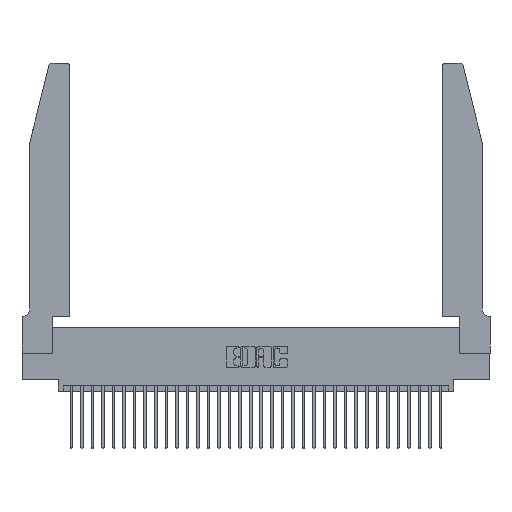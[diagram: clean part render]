
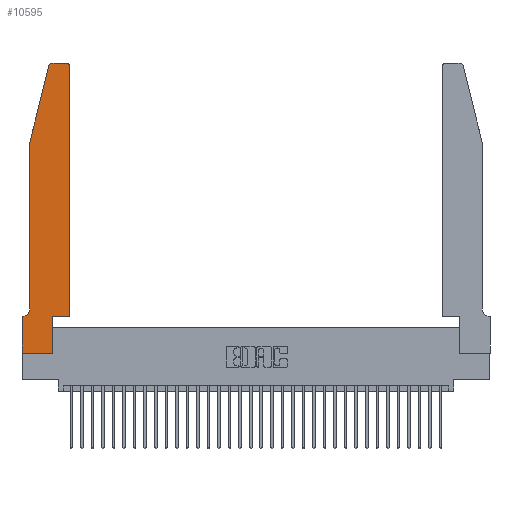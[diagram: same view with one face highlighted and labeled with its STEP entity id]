
A CAD part, top view. The second image highlights one B-rep face of the part: STEP entity #10595.
In plain terms, the highlighted planar face has unit normal (0, 0, 1).
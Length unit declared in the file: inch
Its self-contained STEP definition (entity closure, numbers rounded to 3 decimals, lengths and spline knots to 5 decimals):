
#667 = DIRECTION ( 'NONE',  ( 1., 0., 0. ) ) ;
#1403 = EDGE_CURVE ( 'NONE', #10720, #30104, #23842, .T. ) ;
#1773 = CARTESIAN_POINT ( 'NONE',  ( 0.0055, 0.42, 0.37 ) ) ;
#1906 = VERTEX_POINT ( 'NONE', #26110 ) ;
#2204 = LINE ( 'NONE', #24118, #9197 ) ;
#2300 = ORIENTED_EDGE ( 'NONE', *, *, #12533, .T. ) ;
#2675 = DIRECTION ( 'NONE',  ( 0., 0., 1. ) ) ;
#2886 = ORIENTED_EDGE ( 'NONE', *, *, #8794, .T. ) ;
#3018 = ORIENTED_EDGE ( 'NONE', *, *, #29753, .T. ) ;
#3144 = DIRECTION ( 'NONE',  ( -0.239, -0.971, 0. ) ) ;
#3188 = CIRCLE ( 'NONE', #26327, 0.03 ) ;
#3251 = ORIENTED_EDGE ( 'NONE', *, *, #10801, .T. ) ;
#3457 = VERTEX_POINT ( 'NONE', #25973 ) ;
#4289 = LINE ( 'NONE', #22134, #23551 ) ;
#4416 = DIRECTION ( 'NONE',  ( -1., 0., 0. ) ) ;
#4576 = VECTOR ( 'NONE', #12231, 39.37008 ) ;
#5219 = CARTESIAN_POINT ( 'NONE',  ( 0.4205, 2.75, 0.37 ) ) ;
#5994 = CARTESIAN_POINT ( 'NONE',  ( 0.0755, 0.35, 0.37 ) ) ;
#6241 = EDGE_CURVE ( 'NONE', #12046, #10720, #6479, .T. ) ;
#6479 = LINE ( 'NONE', #24213, #26583 ) ;
#6564 = CARTESIAN_POINT ( 'NONE',  ( 0.4505, 2.72, 0.37 ) ) ;
#6740 = CARTESIAN_POINT ( 'NONE',  ( 0.2865, 0.35, 0.37 ) ) ;
#8004 = LINE ( 'NONE', #16679, #20241 ) ;
#8794 = EDGE_CURVE ( 'NONE', #32573, #12046, #8004, .T. ) ;
#8843 = VECTOR ( 'NONE', #13750, 39.37008 ) ;
#8934 = DIRECTION ( 'NONE',  ( 1., 0., 0. ) ) ;
#9123 = VERTEX_POINT ( 'NONE', #21591 ) ;
#9197 = VECTOR ( 'NONE', #3144, 39.37008 ) ;
#9955 = CARTESIAN_POINT ( 'NONE',  ( 0., 0.35, 0.37 ) ) ;
#10167 = CARTESIAN_POINT ( 'NONE',  ( 0., 0., 0.37 ) ) ;
#10417 = CARTESIAN_POINT ( 'NONE',  ( 0.4505, 0.35, 0.37 ) ) ;
#10595 = ADVANCED_FACE ( 'NONE', ( #31246 ), #19295, .T. ) ;
#10720 = VERTEX_POINT ( 'NONE', #11905 ) ;
#10722 = LINE ( 'NONE', #30584, #4576 ) ;
#10801 = EDGE_CURVE ( 'NONE', #33140, #3457, #10722, .T. ) ;
#11279 = VERTEX_POINT ( 'NONE', #32528 ) ;
#11442 = DIRECTION ( 'NONE',  ( 0., 1., 0. ) ) ;
#11887 = VECTOR ( 'NONE', #17566, 39.37008 ) ;
#11905 = CARTESIAN_POINT ( 'NONE',  ( 0.4505, 0.35, 0.37 ) ) ;
#12046 = VERTEX_POINT ( 'NONE', #6740 ) ;
#12231 = DIRECTION ( 'NONE',  ( -1., 0., 0. ) ) ;
#12533 = EDGE_CURVE ( 'NONE', #29848, #1906, #2204, .T. ) ;
#13750 = DIRECTION ( 'NONE',  ( 0., -1., 0. ) ) ;
#14697 = ORIENTED_EDGE ( 'NONE', *, *, #17729, .T. ) ;
#14990 = EDGE_CURVE ( 'NONE', #1906, #9123, #32786, .T. ) ;
#15049 = DIRECTION ( 'NONE',  ( 0., 1., 0. ) ) ;
#15271 = DIRECTION ( 'NONE',  ( 0., 0., 1. ) ) ;
#15705 = AXIS2_PLACEMENT_3D ( 'NONE', #32400, #24634, #8934 ) ;
#16019 = VECTOR ( 'NONE', #15049, 39.37008 ) ;
#16679 = CARTESIAN_POINT ( 'NONE',  ( 0.2865, 0.35, 0.37 ) ) ;
#16908 = ORIENTED_EDGE ( 'NONE', *, *, #6241, .T. ) ;
#17566 = DIRECTION ( 'NONE',  ( 0., -1., 0. ) ) ;
#17729 = EDGE_CURVE ( 'NONE', #3457, #29848, #29972, .T. ) ;
#17796 = ORIENTED_EDGE ( 'NONE', *, *, #20695, .T. ) ;
#18161 = ORIENTED_EDGE ( 'NONE', *, *, #29936, .T. ) ;
#18311 = CARTESIAN_POINT ( 'NONE',  ( 0.4205, 2.72, 0.37 ) ) ;
#18933 = VERTEX_POINT ( 'NONE', #9955 ) ;
#19030 = CIRCLE ( 'NONE', #31945, 0.07 ) ;
#19295 = PLANE ( 'NONE',  #15705 ) ;
#19907 = EDGE_LOOP ( 'NONE', ( #3251, #14697, #2300, #27234, #23485, #18161, #31059, #17796, #2886, #16908, #25737, #3018 ) ) ;
#20064 = DIRECTION ( 'NONE',  ( 0., 0., -1. ) ) ;
#20169 = EDGE_CURVE ( 'NONE', #9123, #11279, #19030, .T. ) ;
#20188 = CARTESIAN_POINT ( 'NONE',  ( 0.0755, 2., 0.37 ) ) ;
#20241 = VECTOR ( 'NONE', #11442, 39.37008 ) ;
#20695 = EDGE_CURVE ( 'NONE', #27222, #32573, #4289, .T. ) ;
#20959 = DIRECTION ( 'NONE',  ( 1., 0., 0. ) ) ;
#21257 = CARTESIAN_POINT ( 'NONE',  ( 0.2865, 0., 0.37 ) ) ;
#21591 = CARTESIAN_POINT ( 'NONE',  ( 0.0755, 0.42, 0.37 ) ) ;
#21669 = DIRECTION ( 'NONE',  ( -1., 0., 0. ) ) ;
#22134 = CARTESIAN_POINT ( 'NONE',  ( 0., 0., 0.37 ) ) ;
#23485 = ORIENTED_EDGE ( 'NONE', *, *, #20169, .T. ) ;
#23551 = VECTOR ( 'NONE', #30086, 39.37008 ) ;
#23842 = LINE ( 'NONE', #10417, #16019 ) ;
#24118 = CARTESIAN_POINT ( 'NONE',  ( 0.0755, 2., 0.37 ) ) ;
#24213 = CARTESIAN_POINT ( 'NONE',  ( 0.4505, 0.35, 0.37 ) ) ;
#24568 = EDGE_CURVE ( 'NONE', #18933, #27222, #28951, .T. ) ;
#24634 = DIRECTION ( 'NONE',  ( 0., 0., 1. ) ) ;
#25334 = VECTOR ( 'NONE', #21669, 39.37008 ) ;
#25737 = ORIENTED_EDGE ( 'NONE', *, *, #1403, .T. ) ;
#25973 = CARTESIAN_POINT ( 'NONE',  ( 0.284, 2.75, 0.37 ) ) ;
#26110 = CARTESIAN_POINT ( 'NONE',  ( 0.0755, 2., 0.37 ) ) ;
#26149 = LINE ( 'NONE', #5994, #25334 ) ;
#26327 = AXIS2_PLACEMENT_3D ( 'NONE', #18311, #2675, #20959 ) ;
#26583 = VECTOR ( 'NONE', #667, 39.37008 ) ;
#26846 = CARTESIAN_POINT ( 'NONE',  ( 0., 0., 0.37 ) ) ;
#27222 = VERTEX_POINT ( 'NONE', #10167 ) ;
#27234 = ORIENTED_EDGE ( 'NONE', *, *, #14990, .T. ) ;
#27761 = AXIS2_PLACEMENT_3D ( 'NONE', #30988, #15271, #33601 ) ;
#28951 = LINE ( 'NONE', #26846, #8843 ) ;
#29753 = EDGE_CURVE ( 'NONE', #30104, #33140, #3188, .T. ) ;
#29848 = VERTEX_POINT ( 'NONE', #31778 ) ;
#29936 = EDGE_CURVE ( 'NONE', #11279, #18933, #26149, .T. ) ;
#29972 = CIRCLE ( 'NONE', #27761, 0.03 ) ;
#30086 = DIRECTION ( 'NONE',  ( 1., 0., 0. ) ) ;
#30104 = VERTEX_POINT ( 'NONE', #6564 ) ;
#30584 = CARTESIAN_POINT ( 'NONE',  ( 0.2605, 2.75, 0.37 ) ) ;
#30988 = CARTESIAN_POINT ( 'NONE',  ( 0.284, 2.72, 0.37 ) ) ;
#31059 = ORIENTED_EDGE ( 'NONE', *, *, #24568, .T. ) ;
#31246 = FACE_OUTER_BOUND ( 'NONE', #19907, .T. ) ;
#31778 = CARTESIAN_POINT ( 'NONE',  ( 0.25487, 2.72718, 0.37 ) ) ;
#31945 = AXIS2_PLACEMENT_3D ( 'NONE', #1773, #20064, #4416 ) ;
#32400 = CARTESIAN_POINT ( 'NONE',  ( 0., 0.35, 0.37 ) ) ;
#32528 = CARTESIAN_POINT ( 'NONE',  ( 0.0055, 0.35, 0.37 ) ) ;
#32573 = VERTEX_POINT ( 'NONE', #21257 ) ;
#32786 = LINE ( 'NONE', #20188, #11887 ) ;
#33140 = VERTEX_POINT ( 'NONE', #5219 ) ;
#33601 = DIRECTION ( 'NONE',  ( 1., 0., 0. ) ) ;
